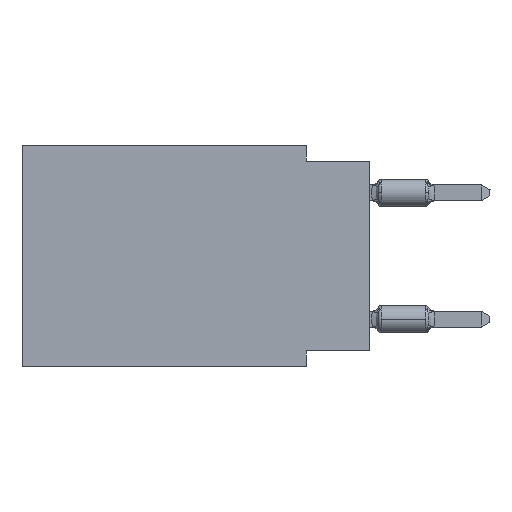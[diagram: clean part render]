
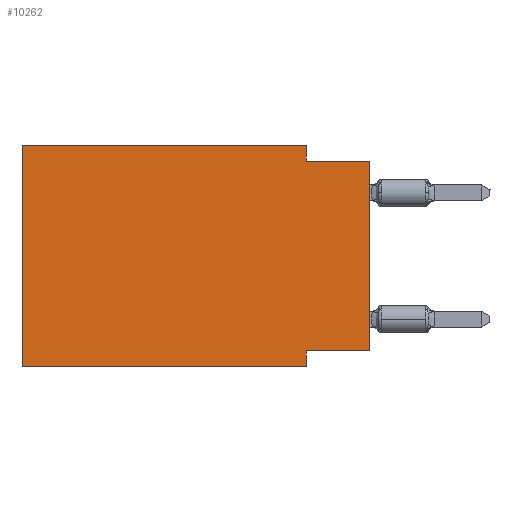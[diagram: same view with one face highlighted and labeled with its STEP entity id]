
A CAD part, left-side view. The second image highlights one B-rep face of the part: STEP entity #10262.
In plain terms, the highlighted planar face has unit normal (-1, 0, 0).
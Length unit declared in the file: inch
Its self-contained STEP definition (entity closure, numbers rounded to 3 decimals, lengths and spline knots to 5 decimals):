
#35 = CARTESIAN_POINT ( 'NONE',  ( 0., 0.55, 0. ) ) ;
#139 = CARTESIAN_POINT ( 'NONE',  ( 0., 0.1, -0.325 ) ) ;
#463 = EDGE_LOOP ( 'NONE', ( #1699, #12377, #10288, #14234, #17733, #17154, #5219, #9788 ) ) ;
#797 = FACE_OUTER_BOUND ( 'NONE', #463, .T. ) ;
#1699 = ORIENTED_EDGE ( 'NONE', *, *, #9502, .T. ) ;
#1823 = EDGE_CURVE ( 'NONE', #5353, #14022, #17947, .T. ) ;
#1978 = VERTEX_POINT ( 'NONE', #17538 ) ;
#2080 = VECTOR ( 'NONE', #14636, 39.37008 ) ;
#2558 = CARTESIAN_POINT ( 'NONE',  ( 0., 0., -0.025 ) ) ;
#2586 = VECTOR ( 'NONE', #4297, 39.37008 ) ;
#3019 = LINE ( 'NONE', #35, #17367 ) ;
#3328 = CARTESIAN_POINT ( 'NONE',  ( 0., 0., -0.325 ) ) ;
#3716 = VECTOR ( 'NONE', #4823, 39.37008 ) ;
#4119 = DIRECTION ( 'NONE',  ( 0., 0., 1. ) ) ;
#4297 = DIRECTION ( 'NONE',  ( 0., 1., 0. ) ) ;
#4408 = VERTEX_POINT ( 'NONE', #18210 ) ;
#4445 = CARTESIAN_POINT ( 'NONE',  ( 0., 0.55, 0. ) ) ;
#4823 = DIRECTION ( 'NONE',  ( 0., -1., 0. ) ) ;
#5219 = ORIENTED_EDGE ( 'NONE', *, *, #12133, .F. ) ;
#5353 = VERTEX_POINT ( 'NONE', #3328 ) ;
#5896 = CARTESIAN_POINT ( 'NONE',  ( 0., 0., -0.325 ) ) ;
#6087 = EDGE_CURVE ( 'NONE', #16962, #19223, #9526, .T. ) ;
#6801 = VECTOR ( 'NONE', #4119, 39.37008 ) ;
#7481 = AXIS2_PLACEMENT_3D ( 'NONE', #14273, #8160, #13070 ) ;
#7569 = CARTESIAN_POINT ( 'NONE',  ( 0., 0.55, 0. ) ) ;
#8133 = CARTESIAN_POINT ( 'NONE',  ( 0., 0.1, -0.35 ) ) ;
#8160 = DIRECTION ( 'NONE',  ( 1., 0., 0. ) ) ;
#8232 = CARTESIAN_POINT ( 'NONE',  ( 0., 0., -0.025 ) ) ;
#8268 = VECTOR ( 'NONE', #18775, 39.37008 ) ;
#8836 = DIRECTION ( 'NONE',  ( 0., -1., 0. ) ) ;
#9212 = LINE ( 'NONE', #9515, #3716 ) ;
#9502 = EDGE_CURVE ( 'NONE', #5353, #13329, #17769, .T. ) ;
#9515 = CARTESIAN_POINT ( 'NONE',  ( 0., 0.55, -0.35 ) ) ;
#9526 = LINE ( 'NONE', #11124, #8268 ) ;
#9743 = CARTESIAN_POINT ( 'NONE',  ( 0., 0.1, -0.025 ) ) ;
#9788 = ORIENTED_EDGE ( 'NONE', *, *, #1823, .F. ) ;
#10262 = ADVANCED_FACE ( 'NONE', ( #797 ), #14570, .F. ) ;
#10263 = DIRECTION ( 'NONE',  ( 0., -1., 0. ) ) ;
#10288 = ORIENTED_EDGE ( 'NONE', *, *, #6087, .F. ) ;
#11082 = EDGE_CURVE ( 'NONE', #4408, #19338, #3019, .T. ) ;
#11124 = CARTESIAN_POINT ( 'NONE',  ( 0., 0.1, 0. ) ) ;
#11308 = CARTESIAN_POINT ( 'NONE',  ( 0., 0., 0. ) ) ;
#11462 = EDGE_CURVE ( 'NONE', #19338, #16962, #17833, .T. ) ;
#11844 = LINE ( 'NONE', #2558, #14563 ) ;
#11965 = CARTESIAN_POINT ( 'NONE',  ( 0., 0.1, 0. ) ) ;
#12133 = EDGE_CURVE ( 'NONE', #14022, #1978, #15723, .T. ) ;
#12377 = ORIENTED_EDGE ( 'NONE', *, *, #18075, .F. ) ;
#13070 = DIRECTION ( 'NONE',  ( 0., 0., -1. ) ) ;
#13329 = VERTEX_POINT ( 'NONE', #8232 ) ;
#14022 = VERTEX_POINT ( 'NONE', #139 ) ;
#14234 = ORIENTED_EDGE ( 'NONE', *, *, #11462, .F. ) ;
#14273 = CARTESIAN_POINT ( 'NONE',  ( 0., 0.55, 0. ) ) ;
#14563 = VECTOR ( 'NONE', #8836, 39.37008 ) ;
#14570 = PLANE ( 'NONE',  #7481 ) ;
#14636 = DIRECTION ( 'NONE',  ( 0., 0., -1. ) ) ;
#15077 = VECTOR ( 'NONE', #10263, 39.37008 ) ;
#15282 = DIRECTION ( 'NONE',  ( 0., 0., 1. ) ) ;
#15723 = LINE ( 'NONE', #8133, #2080 ) ;
#16962 = VERTEX_POINT ( 'NONE', #11965 ) ;
#17154 = ORIENTED_EDGE ( 'NONE', *, *, #18292, .T. ) ;
#17367 = VECTOR ( 'NONE', #15282, 39.37008 ) ;
#17538 = CARTESIAN_POINT ( 'NONE',  ( 0., 0.1, -0.35 ) ) ;
#17733 = ORIENTED_EDGE ( 'NONE', *, *, #11082, .F. ) ;
#17769 = LINE ( 'NONE', #11308, #6801 ) ;
#17833 = LINE ( 'NONE', #7569, #15077 ) ;
#17947 = LINE ( 'NONE', #5896, #2586 ) ;
#18075 = EDGE_CURVE ( 'NONE', #19223, #13329, #11844, .T. ) ;
#18210 = CARTESIAN_POINT ( 'NONE',  ( 0., 0.55, -0.35 ) ) ;
#18292 = EDGE_CURVE ( 'NONE', #4408, #1978, #9212, .T. ) ;
#18775 = DIRECTION ( 'NONE',  ( 0., 0., -1. ) ) ;
#19223 = VERTEX_POINT ( 'NONE', #9743 ) ;
#19338 = VERTEX_POINT ( 'NONE', #4445 ) ;
